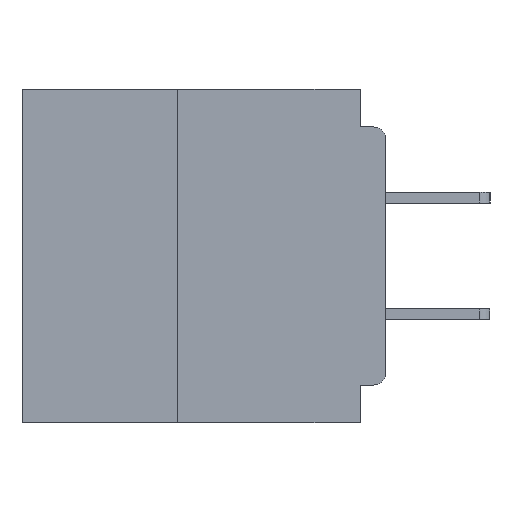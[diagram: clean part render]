
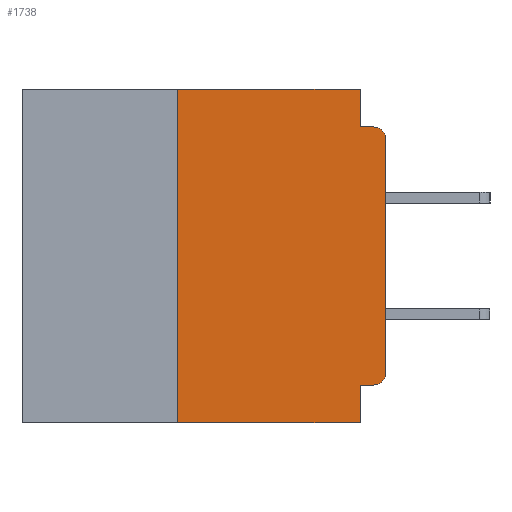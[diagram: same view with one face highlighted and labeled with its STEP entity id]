
A CAD part, left-side view. The second image highlights one B-rep face of the part: STEP entity #1738.
In plain terms, the highlighted planar face has unit normal (-1, 0, 0).
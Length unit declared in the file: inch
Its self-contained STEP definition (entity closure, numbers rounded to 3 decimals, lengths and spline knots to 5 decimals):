
#139 = CARTESIAN_POINT ( 'NONE',  ( 0., 0.031, -0.045 ) ) ;
#428 = VERTEX_POINT ( 'NONE', #24792 ) ;
#562 = DIRECTION ( 'NONE',  ( 0., -1., 0. ) ) ;
#1432 = DIRECTION ( 'NONE',  ( 0., 0., -1. ) ) ;
#1437 = ORIENTED_EDGE ( 'NONE', *, *, #33772, .T. ) ;
#1453 = EDGE_CURVE ( 'NONE', #18742, #7474, #8420, .T. ) ;
#1738 = ADVANCED_FACE ( 'NONE', ( #34878 ), #9953, .F. ) ;
#2218 = ORIENTED_EDGE ( 'NONE', *, *, #10083, .F. ) ;
#3338 = VERTEX_POINT ( 'NONE', #139 ) ;
#3655 = VECTOR ( 'NONE', #35604, 39.37008 ) ;
#3895 = EDGE_CURVE ( 'NONE', #27244, #31340, #10418, .T. ) ;
#3997 = VERTEX_POINT ( 'NONE', #22353 ) ;
#4126 = VECTOR ( 'NONE', #5395, 39.37008 ) ;
#5162 = ORIENTED_EDGE ( 'NONE', *, *, #7679, .T. ) ;
#5239 = VECTOR ( 'NONE', #1432, 39.37008 ) ;
#5278 = CARTESIAN_POINT ( 'NONE',  ( 0., 0.437, 0. ) ) ;
#5395 = DIRECTION ( 'NONE',  ( 0., -1., 0. ) ) ;
#6318 = EDGE_CURVE ( 'NONE', #33021, #18742, #12323, .T. ) ;
#6629 = CARTESIAN_POINT ( 'NONE',  ( 0., 0., 0. ) ) ;
#6699 = CARTESIAN_POINT ( 'NONE',  ( 0., 0., -0.34 ) ) ;
#7474 = VERTEX_POINT ( 'NONE', #12922 ) ;
#7580 = EDGE_CURVE ( 'NONE', #27244, #428, #28892, .T. ) ;
#7679 = EDGE_CURVE ( 'NONE', #13828, #3997, #17999, .T. ) ;
#7756 = ORIENTED_EDGE ( 'NONE', *, *, #1453, .F. ) ;
#8129 = CARTESIAN_POINT ( 'NONE',  ( 0., 0.25, -0.4 ) ) ;
#8420 = LINE ( 'NONE', #18335, #15926 ) ;
#9129 = CARTESIAN_POINT ( 'NONE',  ( 0., 0., -0.045 ) ) ;
#9491 = DIRECTION ( 'NONE',  ( 0., 0., 1. ) ) ;
#9840 = ORIENTED_EDGE ( 'NONE', *, *, #23975, .T. ) ;
#9953 = PLANE ( 'NONE',  #31286 ) ;
#10083 = EDGE_CURVE ( 'NONE', #7474, #3338, #26075, .T. ) ;
#10418 = CIRCLE ( 'NONE', #24534, 0.015 ) ;
#11176 = DIRECTION ( 'NONE',  ( 0., 0., -1. ) ) ;
#11312 = DIRECTION ( 'NONE',  ( -1., 0., 0. ) ) ;
#12323 = LINE ( 'NONE', #8129, #28125 ) ;
#12922 = CARTESIAN_POINT ( 'NONE',  ( 0., 0.031, 0. ) ) ;
#13082 = VERTEX_POINT ( 'NONE', #18871 ) ;
#13483 = CARTESIAN_POINT ( 'NONE',  ( 0., 0.031, 0. ) ) ;
#13647 = DIRECTION ( 'NONE',  ( 0., 1., 0. ) ) ;
#13828 = VERTEX_POINT ( 'NONE', #14628 ) ;
#14109 = LINE ( 'NONE', #9129, #28117 ) ;
#14333 = AXIS2_PLACEMENT_3D ( 'NONE', #28094, #11312, #30889 ) ;
#14628 = CARTESIAN_POINT ( 'NONE',  ( 0., 0., -0.06 ) ) ;
#15177 = CARTESIAN_POINT ( 'NONE',  ( 0., 0.015, -0.355 ) ) ;
#15542 = ORIENTED_EDGE ( 'NONE', *, *, #6318, .F. ) ;
#15838 = ORIENTED_EDGE ( 'NONE', *, *, #36177, .F. ) ;
#15839 = EDGE_LOOP ( 'NONE', ( #1437, #5162, #21477, #2218, #7756, #15542, #9840, #15838, #17411, #19569 ) ) ;
#15926 = VECTOR ( 'NONE', #16766, 39.37008 ) ;
#16766 = DIRECTION ( 'NONE',  ( 0., -1., 0. ) ) ;
#17411 = ORIENTED_EDGE ( 'NONE', *, *, #7580, .F. ) ;
#17999 = CIRCLE ( 'NONE', #14333, 0.015 ) ;
#18335 = CARTESIAN_POINT ( 'NONE',  ( 0., 0.437, 0. ) ) ;
#18742 = VERTEX_POINT ( 'NONE', #32697 ) ;
#18871 = CARTESIAN_POINT ( 'NONE',  ( 0., 0.031, -0.4 ) ) ;
#19569 = ORIENTED_EDGE ( 'NONE', *, *, #3895, .T. ) ;
#19630 = EDGE_CURVE ( 'NONE', #3338, #3997, #14109, .T. ) ;
#20535 = VECTOR ( 'NONE', #13647, 39.37008 ) ;
#21030 = CARTESIAN_POINT ( 'NONE',  ( 0., 0.031, -0.4 ) ) ;
#21057 = LINE ( 'NONE', #21030, #5239 ) ;
#21477 = ORIENTED_EDGE ( 'NONE', *, *, #19630, .F. ) ;
#22353 = CARTESIAN_POINT ( 'NONE',  ( 0., 0.015, -0.045 ) ) ;
#23975 = EDGE_CURVE ( 'NONE', #33021, #13082, #33832, .T. ) ;
#24534 = AXIS2_PLACEMENT_3D ( 'NONE', #26957, #26925, #26913 ) ;
#24792 = CARTESIAN_POINT ( 'NONE',  ( 0., 0.031, -0.355 ) ) ;
#25008 = CARTESIAN_POINT ( 'NONE',  ( 0., 0.437, -0.4 ) ) ;
#25547 = VECTOR ( 'NONE', #9491, 39.37008 ) ;
#26075 = LINE ( 'NONE', #13483, #3655 ) ;
#26301 = CARTESIAN_POINT ( 'NONE',  ( 0., 0.25, -0.4 ) ) ;
#26913 = DIRECTION ( 'NONE',  ( 0., 0., -1. ) ) ;
#26925 = DIRECTION ( 'NONE',  ( -1., 0., 0. ) ) ;
#26957 = CARTESIAN_POINT ( 'NONE',  ( 0., 0.015, -0.34 ) ) ;
#27244 = VERTEX_POINT ( 'NONE', #15177 ) ;
#27695 = DIRECTION ( 'NONE',  ( 0., 0., 1. ) ) ;
#28094 = CARTESIAN_POINT ( 'NONE',  ( 0., 0.015, -0.06 ) ) ;
#28117 = VECTOR ( 'NONE', #562, 39.37008 ) ;
#28125 = VECTOR ( 'NONE', #27695, 39.37008 ) ;
#28892 = LINE ( 'NONE', #35757, #20535 ) ;
#29607 = DIRECTION ( 'NONE',  ( 1., 0., 0. ) ) ;
#30889 = DIRECTION ( 'NONE',  ( 0., 0., -1. ) ) ;
#31286 = AXIS2_PLACEMENT_3D ( 'NONE', #5278, #29607, #11176 ) ;
#31340 = VERTEX_POINT ( 'NONE', #6699 ) ;
#32697 = CARTESIAN_POINT ( 'NONE',  ( 0., 0.25, 0. ) ) ;
#33021 = VERTEX_POINT ( 'NONE', #26301 ) ;
#33755 = LINE ( 'NONE', #6629, #25547 ) ;
#33772 = EDGE_CURVE ( 'NONE', #31340, #13828, #33755, .T. ) ;
#33832 = LINE ( 'NONE', #25008, #4126 ) ;
#34878 = FACE_OUTER_BOUND ( 'NONE', #15839, .T. ) ;
#35604 = DIRECTION ( 'NONE',  ( 0., 0., -1. ) ) ;
#35757 = CARTESIAN_POINT ( 'NONE',  ( 0., 0., -0.355 ) ) ;
#36177 = EDGE_CURVE ( 'NONE', #428, #13082, #21057, .T. ) ;
